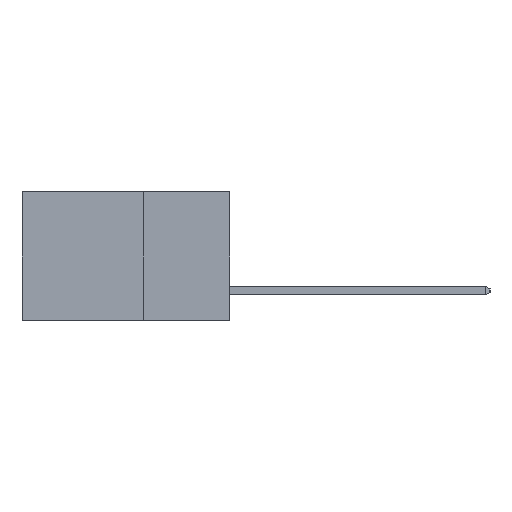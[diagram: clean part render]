
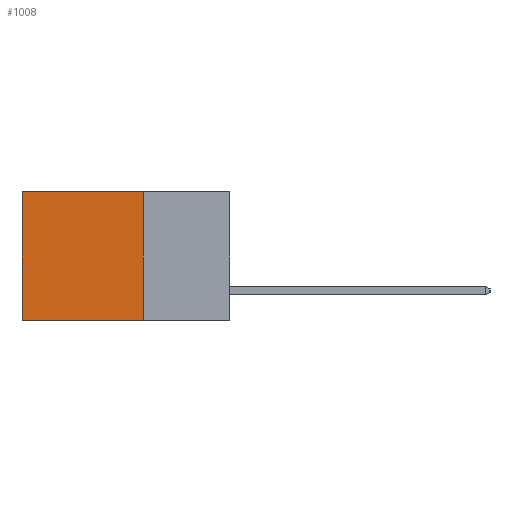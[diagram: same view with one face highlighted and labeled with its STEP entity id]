
A CAD part, left-side view. The second image highlights one B-rep face of the part: STEP entity #1008.
In plain terms, the highlighted planar face has unit normal (-1, 0, 0).
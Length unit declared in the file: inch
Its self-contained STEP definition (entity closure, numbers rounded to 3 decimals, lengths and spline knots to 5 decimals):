
#35 = ORIENTED_EDGE ( 'NONE', *, *, #6255, .F. ) ;
#95 = VECTOR ( 'NONE', #9833, 39.37008 ) ;
#386 = CARTESIAN_POINT ( 'NONE',  ( 0.2615, 0.25, -0.37 ) ) ;
#722 = LINE ( 'NONE', #2245, #95 ) ;
#1008 = ADVANCED_FACE ( 'NONE', ( #9652 ), #7803, .F. ) ;
#1142 = VERTEX_POINT ( 'NONE', #9159 ) ;
#1294 = CARTESIAN_POINT ( 'NONE',  ( 0.2615, 0.25, -0.37 ) ) ;
#1439 = LINE ( 'NONE', #9766, #3484 ) ;
#1776 = VECTOR ( 'NONE', #4697, 39.37008 ) ;
#1863 = EDGE_CURVE ( 'NONE', #4654, #1142, #3739, .T. ) ;
#2245 = CARTESIAN_POINT ( 'NONE',  ( 0.2615, 0.25, 0. ) ) ;
#2617 = EDGE_CURVE ( 'NONE', #3926, #4654, #722, .T. ) ;
#2620 = CARTESIAN_POINT ( 'NONE',  ( 0.2615, 0.25, -0.37 ) ) ;
#2650 = CARTESIAN_POINT ( 'NONE',  ( 0.2615, 0.6, 0. ) ) ;
#3197 = AXIS2_PLACEMENT_3D ( 'NONE', #386, #7838, #7846 ) ;
#3484 = VECTOR ( 'NONE', #3924, 39.37008 ) ;
#3739 = LINE ( 'NONE', #7951, #10383 ) ;
#3924 = DIRECTION ( 'NONE',  ( 0., 0., -1. ) ) ;
#3926 = VERTEX_POINT ( 'NONE', #9904 ) ;
#4151 = VERTEX_POINT ( 'NONE', #2620 ) ;
#4654 = VERTEX_POINT ( 'NONE', #2650 ) ;
#4697 = DIRECTION ( 'NONE',  ( 0., 1., 0. ) ) ;
#5047 = ORIENTED_EDGE ( 'NONE', *, *, #1863, .T. ) ;
#5529 = ORIENTED_EDGE ( 'NONE', *, *, #2617, .T. ) ;
#6255 = EDGE_CURVE ( 'NONE', #3926, #4151, #1439, .T. ) ;
#7803 = PLANE ( 'NONE',  #3197 ) ;
#7831 = EDGE_LOOP ( 'NONE', ( #5047, #9119, #35, #5529 ) ) ;
#7838 = DIRECTION ( 'NONE',  ( 1., 0., 0. ) ) ;
#7846 = DIRECTION ( 'NONE',  ( 0., 0., -1. ) ) ;
#7951 = CARTESIAN_POINT ( 'NONE',  ( 0.2615, 0.6, -0.37 ) ) ;
#8075 = DIRECTION ( 'NONE',  ( 0., 0., -1. ) ) ;
#9119 = ORIENTED_EDGE ( 'NONE', *, *, #10652, .F. ) ;
#9159 = CARTESIAN_POINT ( 'NONE',  ( 0.2615, 0.6, -0.37 ) ) ;
#9652 = FACE_OUTER_BOUND ( 'NONE', #7831, .T. ) ;
#9766 = CARTESIAN_POINT ( 'NONE',  ( 0.2615, 0.25, -0.37 ) ) ;
#9833 = DIRECTION ( 'NONE',  ( 0., 1., 0. ) ) ;
#9904 = CARTESIAN_POINT ( 'NONE',  ( 0.2615, 0.25, 0. ) ) ;
#10383 = VECTOR ( 'NONE', #8075, 39.37008 ) ;
#10438 = LINE ( 'NONE', #1294, #1776 ) ;
#10652 = EDGE_CURVE ( 'NONE', #4151, #1142, #10438, .T. ) ;
